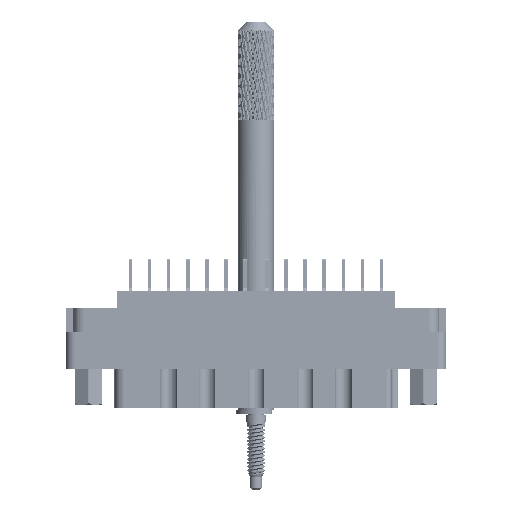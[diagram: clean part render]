
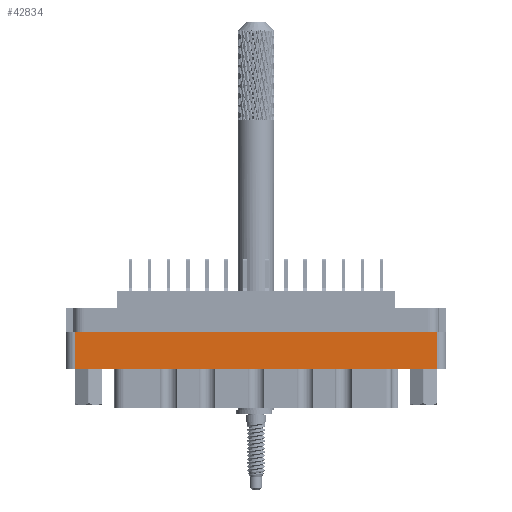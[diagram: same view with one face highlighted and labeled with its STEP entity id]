
A CAD part, front view. The second image highlights one B-rep face of the part: STEP entity #42834.
In plain terms, the highlighted planar face has unit normal (0, -1, 0).
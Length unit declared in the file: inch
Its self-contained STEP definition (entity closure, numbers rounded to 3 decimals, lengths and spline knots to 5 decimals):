
#386 = CARTESIAN_POINT ( 'NONE',  ( 0., -0.438, -0.529 ) ) ;
#1287 = ORIENTED_EDGE ( 'NONE', *, *, #95663, .T. ) ;
#7277 = CARTESIAN_POINT ( 'NONE',  ( -1.234, -0.438, -0.798 ) ) ;
#8915 = CARTESIAN_POINT ( 'NONE',  ( 1.234, -0.438, -0.529 ) ) ;
#22931 = LINE ( 'NONE', #386, #85016 ) ;
#24878 = DIRECTION ( 'NONE',  ( 0., 0., 1. ) ) ;
#25609 = VERTEX_POINT ( 'NONE', #52162 ) ;
#28772 = ORIENTED_EDGE ( 'NONE', *, *, #31306, .T. ) ;
#29464 = EDGE_CURVE ( 'NONE', #25609, #51478, #58119, .T. ) ;
#31306 = EDGE_CURVE ( 'NONE', #85358, #51478, #63823, .T. ) ;
#39013 = CARTESIAN_POINT ( 'NONE',  ( 0., -0.438, -0.277 ) ) ;
#39806 = DIRECTION ( 'NONE',  ( -1., 0., 0. ) ) ;
#42834 = ADVANCED_FACE ( 'NONE', ( #67270 ), #113190, .T. ) ;
#44448 = VECTOR ( 'NONE', #58567, 39.37008 ) ;
#50285 = VERTEX_POINT ( 'NONE', #101767 ) ;
#51478 = VERTEX_POINT ( 'NONE', #55826 ) ;
#52162 = CARTESIAN_POINT ( 'NONE',  ( -1.234, -0.438, -0.277 ) ) ;
#52951 = AXIS2_PLACEMENT_3D ( 'NONE', #94904, #122491, #113586 ) ;
#55826 = CARTESIAN_POINT ( 'NONE',  ( 1.234, -0.438, -0.277 ) ) ;
#56498 = DIRECTION ( 'NONE',  ( 0., 0., -1. ) ) ;
#58119 = LINE ( 'NONE', #39013, #44448 ) ;
#58567 = DIRECTION ( 'NONE',  ( 1., 0., 0. ) ) ;
#59116 = LINE ( 'NONE', #7277, #109180 ) ;
#63823 = LINE ( 'NONE', #112623, #65302 ) ;
#65302 = VECTOR ( 'NONE', #24878, 39.37008 ) ;
#67270 = FACE_OUTER_BOUND ( 'NONE', #80119, .T. ) ;
#80119 = EDGE_LOOP ( 'NONE', ( #105053, #1287, #114268, #28772 ) ) ;
#82741 = EDGE_CURVE ( 'NONE', #85358, #50285, #22931, .T. ) ;
#85016 = VECTOR ( 'NONE', #39806, 39.37008 ) ;
#85358 = VERTEX_POINT ( 'NONE', #8915 ) ;
#94904 = CARTESIAN_POINT ( 'NONE',  ( -1.296, -0.438, -0.798 ) ) ;
#95663 = EDGE_CURVE ( 'NONE', #25609, #50285, #59116, .T. ) ;
#101767 = CARTESIAN_POINT ( 'NONE',  ( -1.234, -0.438, -0.529 ) ) ;
#105053 = ORIENTED_EDGE ( 'NONE', *, *, #29464, .F. ) ;
#109180 = VECTOR ( 'NONE', #56498, 39.37008 ) ;
#112623 = CARTESIAN_POINT ( 'NONE',  ( 1.234, -0.438, -0.798 ) ) ;
#113190 = PLANE ( 'NONE',  #52951 ) ;
#113586 = DIRECTION ( 'NONE',  ( 0., 0., -1. ) ) ;
#114268 = ORIENTED_EDGE ( 'NONE', *, *, #82741, .F. ) ;
#122491 = DIRECTION ( 'NONE',  ( 0., -1., 0. ) ) ;
